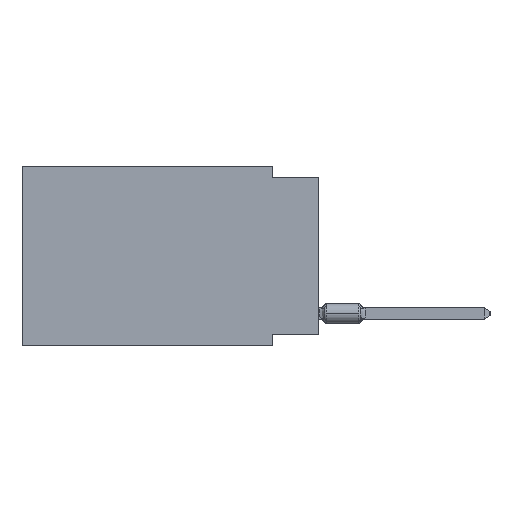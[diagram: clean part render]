
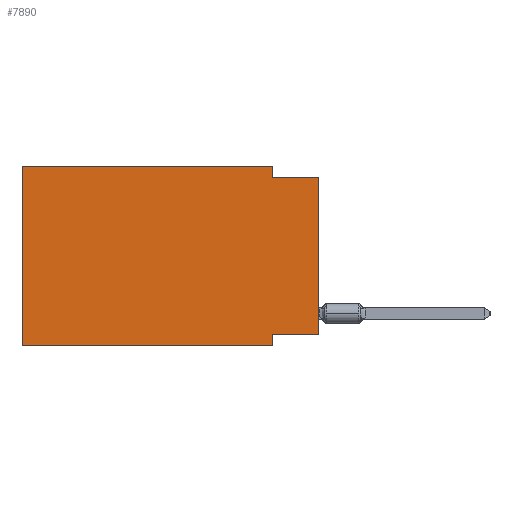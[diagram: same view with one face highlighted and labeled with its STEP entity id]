
A CAD part, left-side view. The second image highlights one B-rep face of the part: STEP entity #7890.
In plain terms, the highlighted planar face has unit normal (-1, 0, 0).
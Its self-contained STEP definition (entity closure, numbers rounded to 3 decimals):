
#77 = EDGE_CURVE ( 'NONE', #21735, #31408, #2518, .T. ) ;
#272 = VECTOR ( 'NONE', #31910, 1000. ) ;
#798 = DIRECTION ( 'NONE',  ( 1., 0., 0. ) ) ;
#1057 = LINE ( 'NONE', #6436, #272 ) ;
#1448 = DIRECTION ( 'NONE',  ( 0., -1., 0. ) ) ;
#2518 = LINE ( 'NONE', #31338, #14331 ) ;
#4145 = VERTEX_POINT ( 'NONE', #19389 ) ;
#4502 = DIRECTION ( 'NONE',  ( 0., -1., 0. ) ) ;
#4840 = LINE ( 'NONE', #15304, #33206 ) ;
#5373 = DIRECTION ( 'NONE',  ( 0., 0., 1. ) ) ;
#6207 = CARTESIAN_POINT ( 'NONE',  ( 0., 2.54, -9.906 ) ) ;
#6436 = CARTESIAN_POINT ( 'NONE',  ( 0., 0., 0. ) ) ;
#6813 = EDGE_LOOP ( 'NONE', ( #19901, #18640, #24747, #16542, #11382, #21257, #12691, #24915 ) ) ;
#6815 = CARTESIAN_POINT ( 'NONE',  ( 0., 2.54, 0. ) ) ;
#7781 = LINE ( 'NONE', #25476, #32552 ) ;
#7890 = ADVANCED_FACE ( 'NONE', ( #23877 ), #26580, .F. ) ;
#8274 = LINE ( 'NONE', #8450, #26546 ) ;
#8375 = VECTOR ( 'NONE', #1448, 1000. ) ;
#8430 = CARTESIAN_POINT ( 'NONE',  ( 0., 0., -9.271 ) ) ;
#8450 = CARTESIAN_POINT ( 'NONE',  ( 0., 2.54, 0. ) ) ;
#10886 = EDGE_CURVE ( 'NONE', #27937, #22345, #8274, .T. ) ;
#10893 = VECTOR ( 'NONE', #5373, 1000. ) ;
#11382 = ORIENTED_EDGE ( 'NONE', *, *, #21569, .F. ) ;
#12353 = VERTEX_POINT ( 'NONE', #16619 ) ;
#12647 = CARTESIAN_POINT ( 'NONE',  ( 0., 16.383, 0. ) ) ;
#12691 = ORIENTED_EDGE ( 'NONE', *, *, #33203, .F. ) ;
#12766 = EDGE_CURVE ( 'NONE', #21735, #4145, #1057, .T. ) ;
#13292 = DIRECTION ( 'NONE',  ( 0., 0., -1. ) ) ;
#14331 = VECTOR ( 'NONE', #31172, 1000. ) ;
#15040 = DIRECTION ( 'NONE',  ( 0., -1., 0. ) ) ;
#15304 = CARTESIAN_POINT ( 'NONE',  ( 0., 0., -0.635 ) ) ;
#16505 = DIRECTION ( 'NONE',  ( 0., 0., -1. ) ) ;
#16542 = ORIENTED_EDGE ( 'NONE', *, *, #30206, .F. ) ;
#16619 = CARTESIAN_POINT ( 'NONE',  ( 0., 2.54, -9.906 ) ) ;
#17998 = VECTOR ( 'NONE', #16505, 1000. ) ;
#18177 = CARTESIAN_POINT ( 'NONE',  ( 0., 16.383, 0. ) ) ;
#18640 = ORIENTED_EDGE ( 'NONE', *, *, #26456, .F. ) ;
#19010 = LINE ( 'NONE', #6207, #17998 ) ;
#19389 = CARTESIAN_POINT ( 'NONE',  ( 0., 0., -0.635 ) ) ;
#19459 = VERTEX_POINT ( 'NONE', #29502 ) ;
#19901 = ORIENTED_EDGE ( 'NONE', *, *, #12766, .T. ) ;
#21257 = ORIENTED_EDGE ( 'NONE', *, *, #29574, .T. ) ;
#21569 = EDGE_CURVE ( 'NONE', #19459, #26731, #30683, .T. ) ;
#21735 = VERTEX_POINT ( 'NONE', #8430 ) ;
#22158 = CARTESIAN_POINT ( 'NONE',  ( 0., 16.383, 0. ) ) ;
#22345 = VERTEX_POINT ( 'NONE', #24359 ) ;
#23877 = FACE_OUTER_BOUND ( 'NONE', #6813, .T. ) ;
#24359 = CARTESIAN_POINT ( 'NONE',  ( 0., 2.54, -0.635 ) ) ;
#24747 = ORIENTED_EDGE ( 'NONE', *, *, #10886, .F. ) ;
#24840 = LINE ( 'NONE', #22158, #8375 ) ;
#24915 = ORIENTED_EDGE ( 'NONE', *, *, #77, .F. ) ;
#25208 = CARTESIAN_POINT ( 'NONE',  ( 0., 2.54, -9.271 ) ) ;
#25476 = CARTESIAN_POINT ( 'NONE',  ( 0., 16.383, -9.906 ) ) ;
#26456 = EDGE_CURVE ( 'NONE', #22345, #4145, #4840, .T. ) ;
#26546 = VECTOR ( 'NONE', #31373, 1000. ) ;
#26580 = PLANE ( 'NONE',  #26859 ) ;
#26731 = VERTEX_POINT ( 'NONE', #32464 ) ;
#26859 = AXIS2_PLACEMENT_3D ( 'NONE', #18177, #798, #13292 ) ;
#27937 = VERTEX_POINT ( 'NONE', #6815 ) ;
#29502 = CARTESIAN_POINT ( 'NONE',  ( 0., 16.383, -9.906 ) ) ;
#29574 = EDGE_CURVE ( 'NONE', #19459, #12353, #7781, .T. ) ;
#30206 = EDGE_CURVE ( 'NONE', #26731, #27937, #24840, .T. ) ;
#30683 = LINE ( 'NONE', #12647, #10893 ) ;
#31172 = DIRECTION ( 'NONE',  ( 0., 1., 0. ) ) ;
#31338 = CARTESIAN_POINT ( 'NONE',  ( 0., 0., -9.271 ) ) ;
#31373 = DIRECTION ( 'NONE',  ( 0., 0., -1. ) ) ;
#31408 = VERTEX_POINT ( 'NONE', #25208 ) ;
#31910 = DIRECTION ( 'NONE',  ( 0., 0., 1. ) ) ;
#32464 = CARTESIAN_POINT ( 'NONE',  ( 0., 16.383, 0. ) ) ;
#32552 = VECTOR ( 'NONE', #15040, 1000. ) ;
#33203 = EDGE_CURVE ( 'NONE', #31408, #12353, #19010, .T. ) ;
#33206 = VECTOR ( 'NONE', #4502, 1000. ) ;
